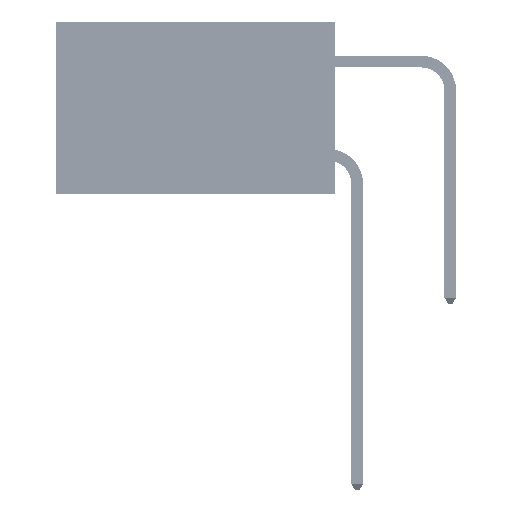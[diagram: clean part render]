
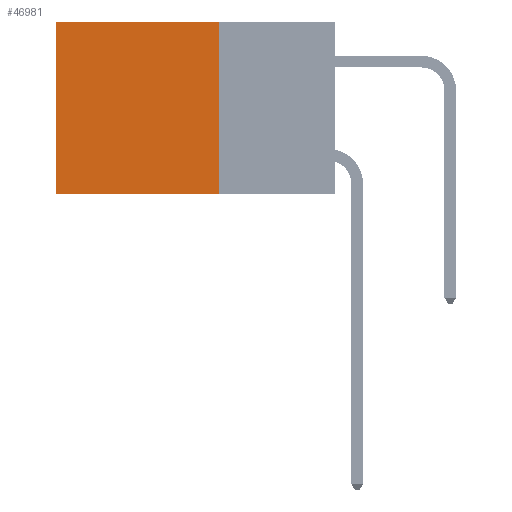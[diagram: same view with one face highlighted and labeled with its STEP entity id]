
A CAD part, left-side view. The second image highlights one B-rep face of the part: STEP entity #46981.
In plain terms, the highlighted planar face has unit normal (-1, 0, 0).
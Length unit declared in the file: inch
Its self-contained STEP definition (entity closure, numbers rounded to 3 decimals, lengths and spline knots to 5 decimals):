
#608 = VECTOR ( 'NONE', #40387, 39.37008 ) ;
#1028 = CARTESIAN_POINT ( 'NONE',  ( 0.2875, 0.25, 0. ) ) ;
#1223 = DIRECTION ( 'NONE',  ( 0., 0., -1. ) ) ;
#3940 = AXIS2_PLACEMENT_3D ( 'NONE', #8272, #36960, #12391 ) ;
#4160 = PLANE ( 'NONE',  #3940 ) ;
#5466 = CARTESIAN_POINT ( 'NONE',  ( 0.2875, 0.25, -0.37 ) ) ;
#5636 = ORIENTED_EDGE ( 'NONE', *, *, #23955, .T. ) ;
#8272 = CARTESIAN_POINT ( 'NONE',  ( 0.2875, 0.25, 0. ) ) ;
#10855 = VERTEX_POINT ( 'NONE', #20152 ) ;
#12391 = DIRECTION ( 'NONE',  ( 0., 0., -1. ) ) ;
#14074 = VECTOR ( 'NONE', #40173, 39.37008 ) ;
#14276 = LINE ( 'NONE', #1028, #33529 ) ;
#15716 = CARTESIAN_POINT ( 'NONE',  ( 0.2875, 0.25, 0. ) ) ;
#17680 = VERTEX_POINT ( 'NONE', #21912 ) ;
#18327 = EDGE_CURVE ( 'NONE', #10855, #40035, #14276, .T. ) ;
#18380 = VERTEX_POINT ( 'NONE', #5466 ) ;
#20143 = EDGE_LOOP ( 'NONE', ( #5636, #49898, #47486, #35032 ) ) ;
#20152 = CARTESIAN_POINT ( 'NONE',  ( 0.2875, 0.25, 0. ) ) ;
#21912 = CARTESIAN_POINT ( 'NONE',  ( 0.2875, 0.6, -0.37 ) ) ;
#22483 = LINE ( 'NONE', #36366, #608 ) ;
#23955 = EDGE_CURVE ( 'NONE', #40035, #17680, #50079, .T. ) ;
#25029 = LINE ( 'NONE', #15716, #14074 ) ;
#33529 = VECTOR ( 'NONE', #49932, 39.37008 ) ;
#35032 = ORIENTED_EDGE ( 'NONE', *, *, #18327, .T. ) ;
#36366 = CARTESIAN_POINT ( 'NONE',  ( 0.2875, 0.25, -0.37 ) ) ;
#36960 = DIRECTION ( 'NONE',  ( 1., 0., 0. ) ) ;
#37912 = CARTESIAN_POINT ( 'NONE',  ( 0.2875, 0.6, 0. ) ) ;
#39315 = VECTOR ( 'NONE', #1223, 39.37008 ) ;
#40035 = VERTEX_POINT ( 'NONE', #41730 ) ;
#40173 = DIRECTION ( 'NONE',  ( 0., 0., -1. ) ) ;
#40387 = DIRECTION ( 'NONE',  ( 0., 1., 0. ) ) ;
#41730 = CARTESIAN_POINT ( 'NONE',  ( 0.2875, 0.6, 0. ) ) ;
#46981 = ADVANCED_FACE ( 'NONE', ( #51199 ), #4160, .F. ) ;
#47486 = ORIENTED_EDGE ( 'NONE', *, *, #48211, .F. ) ;
#48211 = EDGE_CURVE ( 'NONE', #10855, #18380, #25029, .T. ) ;
#48918 = EDGE_CURVE ( 'NONE', #18380, #17680, #22483, .T. ) ;
#49898 = ORIENTED_EDGE ( 'NONE', *, *, #48918, .F. ) ;
#49932 = DIRECTION ( 'NONE',  ( 0., 1., 0. ) ) ;
#50079 = LINE ( 'NONE', #37912, #39315 ) ;
#51199 = FACE_OUTER_BOUND ( 'NONE', #20143, .T. ) ;
